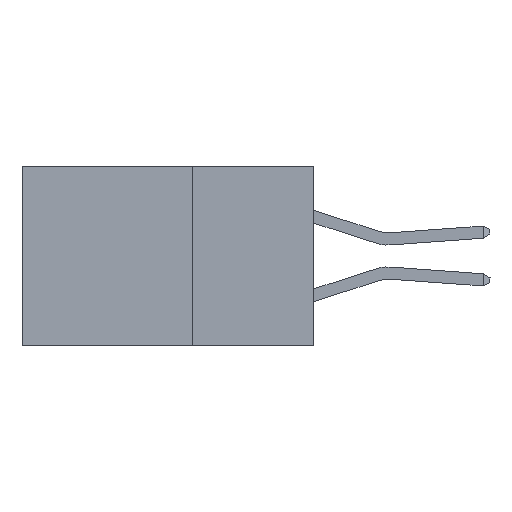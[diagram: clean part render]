
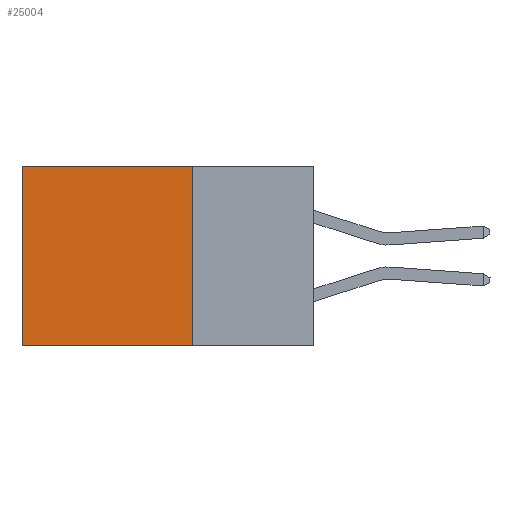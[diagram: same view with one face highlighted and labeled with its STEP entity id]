
A CAD part, left-side view. The second image highlights one B-rep face of the part: STEP entity #25004.
In plain terms, the highlighted planar face has unit normal (-1, 0, 0).
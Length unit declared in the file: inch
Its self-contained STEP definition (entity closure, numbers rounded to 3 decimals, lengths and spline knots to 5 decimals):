
#151 = CARTESIAN_POINT ( 'NONE',  ( 0.2875, 0.25, 0. ) ) ;
#254 = LINE ( 'NONE', #151, #27222 ) ;
#459 = DIRECTION ( 'NONE',  ( 0., 0., -1. ) ) ;
#589 = ORIENTED_EDGE ( 'NONE', *, *, #13723, .F. ) ;
#2989 = VECTOR ( 'NONE', #19626, 39.37008 ) ;
#3594 = CARTESIAN_POINT ( 'NONE',  ( 0.2875, 0.25, -0.37 ) ) ;
#4349 = EDGE_CURVE ( 'NONE', #17519, #27291, #28596, .T. ) ;
#5136 = EDGE_LOOP ( 'NONE', ( #22405, #589, #27512, #9508 ) ) ;
#7519 = DIRECTION ( 'NONE',  ( 0., 0., -1. ) ) ;
#7966 = DIRECTION ( 'NONE',  ( 0., 1., 0. ) ) ;
#8100 = VECTOR ( 'NONE', #7966, 39.37008 ) ;
#8777 = LINE ( 'NONE', #3594, #2989 ) ;
#9508 = ORIENTED_EDGE ( 'NONE', *, *, #4349, .T. ) ;
#9786 = DIRECTION ( 'NONE',  ( 0., 0., -1. ) ) ;
#11601 = CARTESIAN_POINT ( 'NONE',  ( 0.2875, 0.25, 0. ) ) ;
#11811 = DIRECTION ( 'NONE',  ( 1., 0., 0. ) ) ;
#12465 = VERTEX_POINT ( 'NONE', #19943 ) ;
#12590 = VECTOR ( 'NONE', #7519, 39.37008 ) ;
#13723 = EDGE_CURVE ( 'NONE', #24127, #12465, #8777, .T. ) ;
#16551 = EDGE_CURVE ( 'NONE', #17519, #24127, #254, .T. ) ;
#16874 = CARTESIAN_POINT ( 'NONE',  ( 0.2875, 0.25, 0. ) ) ;
#17150 = FACE_OUTER_BOUND ( 'NONE', #5136, .T. ) ;
#17519 = VERTEX_POINT ( 'NONE', #21824 ) ;
#19626 = DIRECTION ( 'NONE',  ( 0., 1., 0. ) ) ;
#19943 = CARTESIAN_POINT ( 'NONE',  ( 0.2875, 0.6, -0.37 ) ) ;
#20020 = AXIS2_PLACEMENT_3D ( 'NONE', #11601, #11811, #9786 ) ;
#21044 = CARTESIAN_POINT ( 'NONE',  ( 0.2875, 0.6, 0. ) ) ;
#21824 = CARTESIAN_POINT ( 'NONE',  ( 0.2875, 0.25, 0. ) ) ;
#21873 = LINE ( 'NONE', #21044, #12590 ) ;
#22405 = ORIENTED_EDGE ( 'NONE', *, *, #23977, .T. ) ;
#22921 = PLANE ( 'NONE',  #20020 ) ;
#23851 = CARTESIAN_POINT ( 'NONE',  ( 0.2875, 0.6, 0. ) ) ;
#23977 = EDGE_CURVE ( 'NONE', #27291, #12465, #21873, .T. ) ;
#24127 = VERTEX_POINT ( 'NONE', #28644 ) ;
#25004 = ADVANCED_FACE ( 'NONE', ( #17150 ), #22921, .F. ) ;
#27222 = VECTOR ( 'NONE', #459, 39.37008 ) ;
#27291 = VERTEX_POINT ( 'NONE', #23851 ) ;
#27512 = ORIENTED_EDGE ( 'NONE', *, *, #16551, .F. ) ;
#28596 = LINE ( 'NONE', #16874, #8100 ) ;
#28644 = CARTESIAN_POINT ( 'NONE',  ( 0.2875, 0.25, -0.37 ) ) ;
